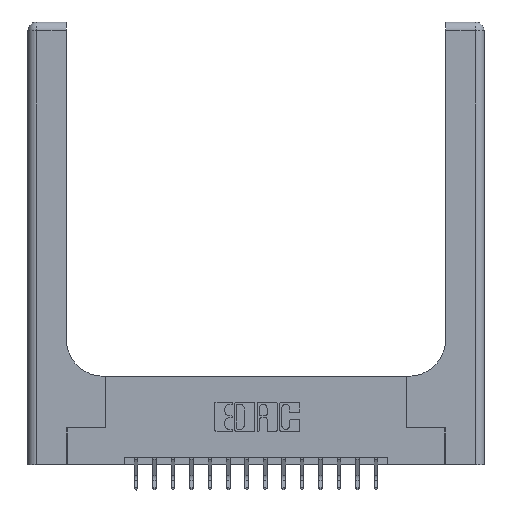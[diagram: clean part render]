
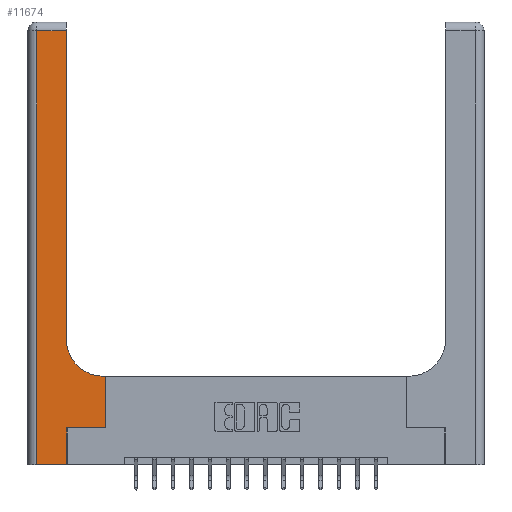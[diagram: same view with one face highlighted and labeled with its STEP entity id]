
A CAD part, top view. The second image highlights one B-rep face of the part: STEP entity #11674.
In plain terms, the highlighted planar face has unit normal (0, 0, 1).
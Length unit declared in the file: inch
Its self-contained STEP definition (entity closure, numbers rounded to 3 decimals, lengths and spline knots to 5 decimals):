
#208 = CARTESIAN_POINT ( 'NONE',  ( 0.265, 0., 0.37 ) ) ;
#595 = DIRECTION ( 'NONE',  ( 1., 0., 0. ) ) ;
#740 = ORIENTED_EDGE ( 'NONE', *, *, #11186, .T. ) ;
#742 = VERTEX_POINT ( 'NONE', #8348 ) ;
#744 = DIRECTION ( 'NONE',  ( 0., 1., 0. ) ) ;
#981 = CARTESIAN_POINT ( 'NONE',  ( 0.26, 0.85, 0.37 ) ) ;
#1049 = CARTESIAN_POINT ( 'NONE',  ( 0.06, 2.94, 0.37 ) ) ;
#1769 = EDGE_CURVE ( 'NONE', #11627, #14577, #10528, .T. ) ;
#1828 = CARTESIAN_POINT ( 'NONE',  ( 0.26, 2.94, 0.37 ) ) ;
#1952 = ORIENTED_EDGE ( 'NONE', *, *, #9281, .T. ) ;
#2069 = CARTESIAN_POINT ( 'NONE',  ( 0.265, 0.25, 0.37 ) ) ;
#2354 = LINE ( 'NONE', #16351, #7154 ) ;
#2819 = VERTEX_POINT ( 'NONE', #1828 ) ;
#3122 = VERTEX_POINT ( 'NONE', #1049 ) ;
#3239 = ORIENTED_EDGE ( 'NONE', *, *, #17608, .T. ) ;
#3350 = DIRECTION ( 'NONE',  ( 1., 0., 0. ) ) ;
#3469 = DIRECTION ( 'NONE',  ( 0., 0., -1. ) ) ;
#3700 = CARTESIAN_POINT ( 'NONE',  ( 0.528, 0.25, 0.37 ) ) ;
#4475 = LINE ( 'NONE', #9096, #7777 ) ;
#4496 = CARTESIAN_POINT ( 'NONE',  ( 0., 0., 0.37 ) ) ;
#5290 = ORIENTED_EDGE ( 'NONE', *, *, #5761, .T. ) ;
#5576 = VERTEX_POINT ( 'NONE', #7301 ) ;
#5761 = EDGE_CURVE ( 'NONE', #14577, #5576, #16163, .T. ) ;
#6055 = ORIENTED_EDGE ( 'NONE', *, *, #16199, .T. ) ;
#6142 = EDGE_CURVE ( 'NONE', #742, #10964, #13268, .T. ) ;
#6634 = EDGE_LOOP ( 'NONE', ( #3239, #1952, #740, #7488, #6055, #11584, #5290, #8601, #15073 ) ) ;
#6934 = LINE ( 'NONE', #7842, #13130 ) ;
#7154 = VECTOR ( 'NONE', #17828, 39.37008 ) ;
#7301 = CARTESIAN_POINT ( 'NONE',  ( 0.528, 0.6, 0.37 ) ) ;
#7488 = ORIENTED_EDGE ( 'NONE', *, *, #6142, .T. ) ;
#7579 = DIRECTION ( 'NONE',  ( -1., 0., 0. ) ) ;
#7613 = DIRECTION ( 'NONE',  ( 0., 0., -1. ) ) ;
#7777 = VECTOR ( 'NONE', #744, 39.37008 ) ;
#7842 = CARTESIAN_POINT ( 'NONE',  ( 0., 2.94, 0.37 ) ) ;
#7909 = DIRECTION ( 'NONE',  ( -1., 0., 0. ) ) ;
#8030 = CARTESIAN_POINT ( 'NONE',  ( 0.26, 0.6, 0.37 ) ) ;
#8348 = CARTESIAN_POINT ( 'NONE',  ( 0.06, 0., 0.37 ) ) ;
#8550 = AXIS2_PLACEMENT_3D ( 'NONE', #16090, #3469, #7579 ) ;
#8601 = ORIENTED_EDGE ( 'NONE', *, *, #15582, .T. ) ;
#9034 = VECTOR ( 'NONE', #10270, 39.37008 ) ;
#9096 = CARTESIAN_POINT ( 'NONE',  ( 0.26, 3., 0.37 ) ) ;
#9177 = LINE ( 'NONE', #10989, #13633 ) ;
#9281 = EDGE_CURVE ( 'NONE', #2819, #3122, #6934, .T. ) ;
#9669 = VECTOR ( 'NONE', #3350, 39.37008 ) ;
#9989 = FACE_OUTER_BOUND ( 'NONE', #6634, .T. ) ;
#10270 = DIRECTION ( 'NONE',  ( 0., 1., 0. ) ) ;
#10289 = VECTOR ( 'NONE', #7909, 39.37008 ) ;
#10528 = LINE ( 'NONE', #11329, #9669 ) ;
#10888 = DIRECTION ( 'NONE',  ( -1., 0., 0. ) ) ;
#10964 = VERTEX_POINT ( 'NONE', #208 ) ;
#10989 = CARTESIAN_POINT ( 'NONE',  ( 0.265, 0., 0.37 ) ) ;
#11186 = EDGE_CURVE ( 'NONE', #3122, #742, #2354, .T. ) ;
#11329 = CARTESIAN_POINT ( 'NONE',  ( 0.265, 0.25, 0.37 ) ) ;
#11584 = ORIENTED_EDGE ( 'NONE', *, *, #1769, .T. ) ;
#11627 = VERTEX_POINT ( 'NONE', #2069 ) ;
#11674 = ADVANCED_FACE ( 'NONE', ( #9989 ), #14668, .F. ) ;
#13130 = VECTOR ( 'NONE', #10888, 39.37008 ) ;
#13268 = LINE ( 'NONE', #4496, #17246 ) ;
#13633 = VECTOR ( 'NONE', #15437, 39.37008 ) ;
#13748 = VERTEX_POINT ( 'NONE', #981 ) ;
#13901 = AXIS2_PLACEMENT_3D ( 'NONE', #14576, #7613, #595 ) ;
#13932 = EDGE_CURVE ( 'NONE', #14064, #13748, #15496, .T. ) ;
#13997 = CARTESIAN_POINT ( 'NONE',  ( 0.51, 0.6, 0.37 ) ) ;
#14064 = VERTEX_POINT ( 'NONE', #13997 ) ;
#14576 = CARTESIAN_POINT ( 'NONE',  ( 0.51, 0.85, 0.37 ) ) ;
#14577 = VERTEX_POINT ( 'NONE', #3700 ) ;
#14668 = PLANE ( 'NONE',  #8550 ) ;
#15073 = ORIENTED_EDGE ( 'NONE', *, *, #13932, .T. ) ;
#15437 = DIRECTION ( 'NONE',  ( 0., 1., 0. ) ) ;
#15496 = CIRCLE ( 'NONE', #13901, 0.25 ) ;
#15582 = EDGE_CURVE ( 'NONE', #5576, #14064, #17875, .T. ) ;
#15756 = DIRECTION ( 'NONE',  ( 1., 0., 0. ) ) ;
#16090 = CARTESIAN_POINT ( 'NONE',  ( 0., 3., 0.37 ) ) ;
#16163 = LINE ( 'NONE', #16393, #9034 ) ;
#16199 = EDGE_CURVE ( 'NONE', #10964, #11627, #9177, .T. ) ;
#16351 = CARTESIAN_POINT ( 'NONE',  ( 0.06, 3., 0.37 ) ) ;
#16393 = CARTESIAN_POINT ( 'NONE',  ( 0.528, 0.25, 0.37 ) ) ;
#17246 = VECTOR ( 'NONE', #15756, 39.37008 ) ;
#17608 = EDGE_CURVE ( 'NONE', #13748, #2819, #4475, .T. ) ;
#17828 = DIRECTION ( 'NONE',  ( 0., -1., 0. ) ) ;
#17875 = LINE ( 'NONE', #8030, #10289 ) ;
